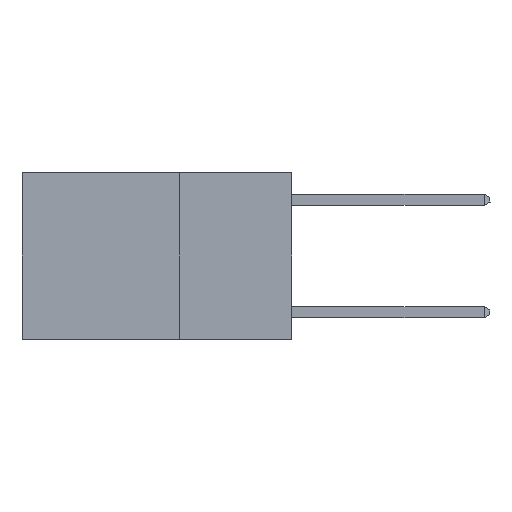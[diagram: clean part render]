
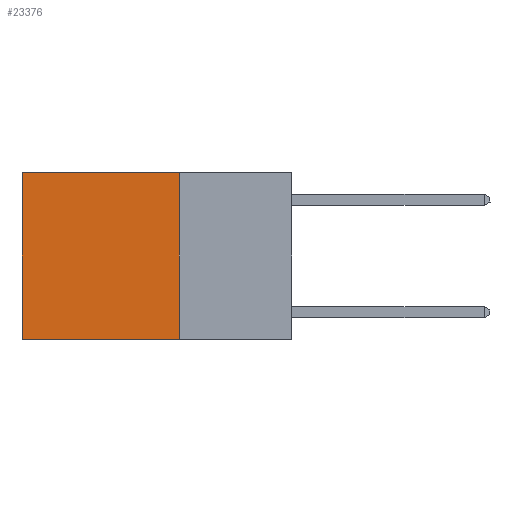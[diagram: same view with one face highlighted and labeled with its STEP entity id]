
A CAD part, left-side view. The second image highlights one B-rep face of the part: STEP entity #23376.
In plain terms, the highlighted planar face has unit normal (-1, 0, 0).
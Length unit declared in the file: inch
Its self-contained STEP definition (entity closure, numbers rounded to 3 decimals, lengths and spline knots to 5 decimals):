
#1557 = VECTOR ( 'NONE', #7694, 39.37008 ) ;
#1759 = CARTESIAN_POINT ( 'NONE',  ( 0.2625, 0.6, 0. ) ) ;
#2899 = VERTEX_POINT ( 'NONE', #25343 ) ;
#3465 = EDGE_CURVE ( 'NONE', #16786, #2899, #11155, .T. ) ;
#3527 = CARTESIAN_POINT ( 'NONE',  ( 0.2625, 0.25, -0.37 ) ) ;
#3883 = EDGE_CURVE ( 'NONE', #7349, #11643, #10559, .T. ) ;
#4998 = LINE ( 'NONE', #16521, #1557 ) ;
#6074 = EDGE_CURVE ( 'NONE', #7349, #16786, #4998, .T. ) ;
#6150 = CARTESIAN_POINT ( 'NONE',  ( 0.2625, 0.25, -0.37 ) ) ;
#6835 = ORIENTED_EDGE ( 'NONE', *, *, #3883, .F. ) ;
#6842 = ORIENTED_EDGE ( 'NONE', *, *, #6074, .T. ) ;
#7349 = VERTEX_POINT ( 'NONE', #8402 ) ;
#7694 = DIRECTION ( 'NONE',  ( 0., 1., 0. ) ) ;
#8279 = CARTESIAN_POINT ( 'NONE',  ( 0.2625, 0.6, 0. ) ) ;
#8402 = CARTESIAN_POINT ( 'NONE',  ( 0.2625, 0.25, 0. ) ) ;
#8742 = VECTOR ( 'NONE', #12600, 39.37008 ) ;
#8747 = VECTOR ( 'NONE', #10481, 39.37008 ) ;
#9450 = ORIENTED_EDGE ( 'NONE', *, *, #3465, .T. ) ;
#10481 = DIRECTION ( 'NONE',  ( 0., 0., -1. ) ) ;
#10559 = LINE ( 'NONE', #11101, #23023 ) ;
#11101 = CARTESIAN_POINT ( 'NONE',  ( 0.2625, 0.25, 0. ) ) ;
#11155 = LINE ( 'NONE', #8279, #8747 ) ;
#11643 = VERTEX_POINT ( 'NONE', #3527 ) ;
#11783 = AXIS2_PLACEMENT_3D ( 'NONE', #16734, #25595, #18770 ) ;
#12600 = DIRECTION ( 'NONE',  ( 0., 1., 0. ) ) ;
#15049 = EDGE_CURVE ( 'NONE', #11643, #2899, #28476, .T. ) ;
#15974 = ORIENTED_EDGE ( 'NONE', *, *, #15049, .F. ) ;
#16521 = CARTESIAN_POINT ( 'NONE',  ( 0.2625, 0.25, 0. ) ) ;
#16734 = CARTESIAN_POINT ( 'NONE',  ( 0.2625, 0.25, 0. ) ) ;
#16786 = VERTEX_POINT ( 'NONE', #1759 ) ;
#17469 = FACE_OUTER_BOUND ( 'NONE', #19782, .T. ) ;
#18770 = DIRECTION ( 'NONE',  ( 0., 0., -1. ) ) ;
#19782 = EDGE_LOOP ( 'NONE', ( #9450, #15974, #6835, #6842 ) ) ;
#23023 = VECTOR ( 'NONE', #24717, 39.37008 ) ;
#23376 = ADVANCED_FACE ( 'NONE', ( #17469 ), #27537, .F. ) ;
#24717 = DIRECTION ( 'NONE',  ( 0., 0., -1. ) ) ;
#25343 = CARTESIAN_POINT ( 'NONE',  ( 0.2625, 0.6, -0.37 ) ) ;
#25595 = DIRECTION ( 'NONE',  ( 1., 0., 0. ) ) ;
#27537 = PLANE ( 'NONE',  #11783 ) ;
#28476 = LINE ( 'NONE', #6150, #8742 ) ;
